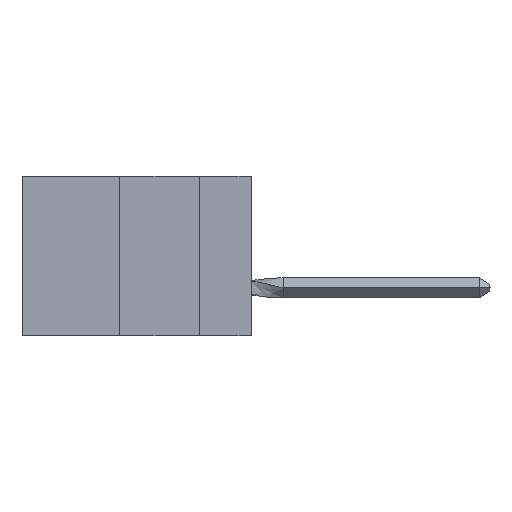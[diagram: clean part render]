
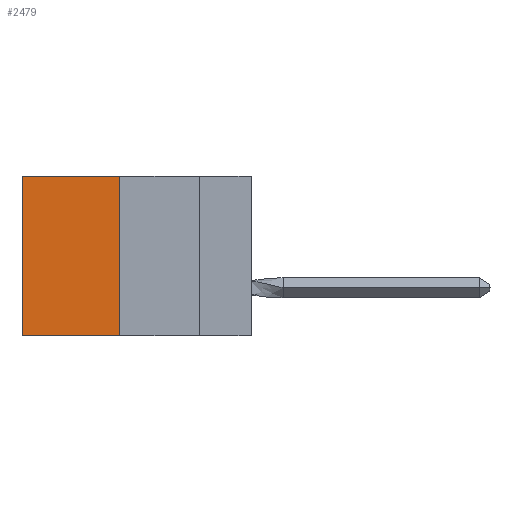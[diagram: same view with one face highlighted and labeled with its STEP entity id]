
A CAD part, left-side view. The second image highlights one B-rep face of the part: STEP entity #2479.
In plain terms, the highlighted planar face has unit normal (-1, 0, 0).
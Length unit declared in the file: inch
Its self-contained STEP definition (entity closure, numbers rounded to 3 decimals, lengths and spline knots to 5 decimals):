
#394 = CARTESIAN_POINT ( 'NONE',  ( 0.305, 0.413, -0.5 ) ) ;
#1001 = EDGE_CURVE ( 'NONE', #15904, #18078, #26506, .T. ) ;
#2104 = VECTOR ( 'NONE', #11846, 39.37008 ) ;
#2292 = ORIENTED_EDGE ( 'NONE', *, *, #11669, .F. ) ;
#2479 = ADVANCED_FACE ( 'NONE', ( #16967 ), #6557, .F. ) ;
#3960 = DIRECTION ( 'NONE',  ( 0., 0., -1. ) ) ;
#4366 = VERTEX_POINT ( 'NONE', #28406 ) ;
#4549 = VECTOR ( 'NONE', #8674, 39.37008 ) ;
#5445 = CARTESIAN_POINT ( 'NONE',  ( 0.305, 0.413, -0.5 ) ) ;
#6270 = CARTESIAN_POINT ( 'NONE',  ( 0.305, 0.413, 0. ) ) ;
#6504 = VERTEX_POINT ( 'NONE', #12989 ) ;
#6557 = PLANE ( 'NONE',  #28273 ) ;
#6816 = LINE ( 'NONE', #6270, #7216 ) ;
#7216 = VECTOR ( 'NONE', #13807, 39.37008 ) ;
#7664 = DIRECTION ( 'NONE',  ( 0., 0., -1. ) ) ;
#8298 = EDGE_LOOP ( 'NONE', ( #25462, #16978, #2292, #15670 ) ) ;
#8674 = DIRECTION ( 'NONE',  ( 0., 0., -1. ) ) ;
#11669 = EDGE_CURVE ( 'NONE', #4366, #15904, #13727, .T. ) ;
#11846 = DIRECTION ( 'NONE',  ( 0., 1., 0. ) ) ;
#12989 = CARTESIAN_POINT ( 'NONE',  ( 0.305, 0.72, 0. ) ) ;
#13727 = LINE ( 'NONE', #394, #29673 ) ;
#13807 = DIRECTION ( 'NONE',  ( 0., 1., 0. ) ) ;
#15670 = ORIENTED_EDGE ( 'NONE', *, *, #21082, .T. ) ;
#15904 = VERTEX_POINT ( 'NONE', #5445 ) ;
#16495 = DIRECTION ( 'NONE',  ( 1., 0., 0. ) ) ;
#16967 = FACE_OUTER_BOUND ( 'NONE', #8298, .T. ) ;
#16978 = ORIENTED_EDGE ( 'NONE', *, *, #1001, .F. ) ;
#18078 = VERTEX_POINT ( 'NONE', #31422 ) ;
#18297 = CARTESIAN_POINT ( 'NONE',  ( 0.305, 0.72, -0.5 ) ) ;
#20202 = LINE ( 'NONE', #18297, #4549 ) ;
#21082 = EDGE_CURVE ( 'NONE', #4366, #6504, #6816, .T. ) ;
#24075 = CARTESIAN_POINT ( 'NONE',  ( 0.305, 0.413, -0.5 ) ) ;
#25462 = ORIENTED_EDGE ( 'NONE', *, *, #28137, .T. ) ;
#26135 = CARTESIAN_POINT ( 'NONE',  ( 0.305, 0.413, -0.5 ) ) ;
#26506 = LINE ( 'NONE', #24075, #2104 ) ;
#28137 = EDGE_CURVE ( 'NONE', #6504, #18078, #20202, .T. ) ;
#28273 = AXIS2_PLACEMENT_3D ( 'NONE', #26135, #16495, #3960 ) ;
#28406 = CARTESIAN_POINT ( 'NONE',  ( 0.305, 0.413, 0. ) ) ;
#29673 = VECTOR ( 'NONE', #7664, 39.37008 ) ;
#31422 = CARTESIAN_POINT ( 'NONE',  ( 0.305, 0.72, -0.5 ) ) ;
